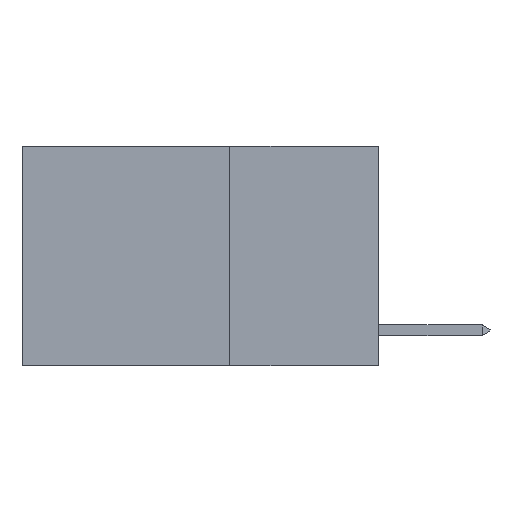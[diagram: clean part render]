
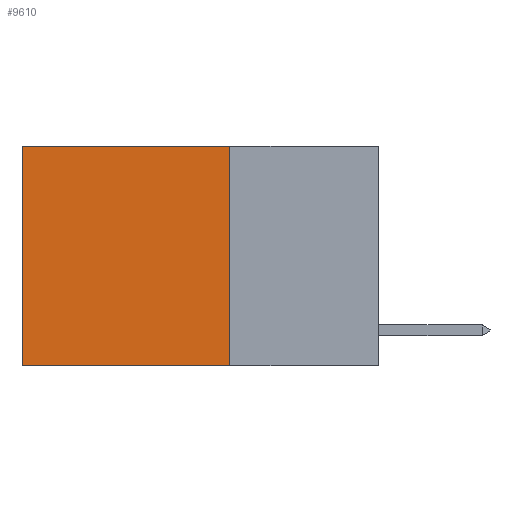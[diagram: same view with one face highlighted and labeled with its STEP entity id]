
A CAD part, left-side view. The second image highlights one B-rep face of the part: STEP entity #9610.
In plain terms, the highlighted planar face has unit normal (-1, 0, 0).
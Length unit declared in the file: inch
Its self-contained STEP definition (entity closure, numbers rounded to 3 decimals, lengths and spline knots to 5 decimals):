
#3048 = CARTESIAN_POINT ( 'NONE',  ( 0.2625, 0.6, -0.37 ) ) ;
#3465 = VECTOR ( 'NONE', #12344, 39.37008 ) ;
#3914 = CARTESIAN_POINT ( 'NONE',  ( 0.2625, 0.25, -0.37 ) ) ;
#4142 = EDGE_CURVE ( 'NONE', #28734, #22519, #23128, .T. ) ;
#4791 = DIRECTION ( 'NONE',  ( 0., 1., 0. ) ) ;
#5929 = CARTESIAN_POINT ( 'NONE',  ( 0.2625, 0.25, 0. ) ) ;
#8169 = VECTOR ( 'NONE', #30940, 39.37008 ) ;
#8349 = DIRECTION ( 'NONE',  ( 0., 0., -1. ) ) ;
#8945 = LINE ( 'NONE', #26161, #8169 ) ;
#9506 = VERTEX_POINT ( 'NONE', #3048 ) ;
#9610 = ADVANCED_FACE ( 'NONE', ( #30795 ), #17893, .F. ) ;
#9884 = LINE ( 'NONE', #14764, #3465 ) ;
#10461 = AXIS2_PLACEMENT_3D ( 'NONE', #5929, #22759, #8349 ) ;
#12344 = DIRECTION ( 'NONE',  ( 0., 0., -1. ) ) ;
#12911 = ORIENTED_EDGE ( 'NONE', *, *, #28765, .T. ) ;
#13564 = EDGE_CURVE ( 'NONE', #29438, #9506, #20241, .T. ) ;
#14479 = CARTESIAN_POINT ( 'NONE',  ( 0.2625, 0.25, -0.37 ) ) ;
#14650 = DIRECTION ( 'NONE',  ( 0., 1., 0. ) ) ;
#14764 = CARTESIAN_POINT ( 'NONE',  ( 0.2625, 0.6, 0. ) ) ;
#15971 = VECTOR ( 'NONE', #14650, 39.37008 ) ;
#17893 = PLANE ( 'NONE',  #10461 ) ;
#17933 = ORIENTED_EDGE ( 'NONE', *, *, #4142, .T. ) ;
#18714 = VECTOR ( 'NONE', #4791, 39.37008 ) ;
#19484 = CARTESIAN_POINT ( 'NONE',  ( 0.2625, 0.25, 0. ) ) ;
#19889 = CARTESIAN_POINT ( 'NONE',  ( 0.2625, 0.6, 0. ) ) ;
#20241 = LINE ( 'NONE', #14479, #18714 ) ;
#22519 = VERTEX_POINT ( 'NONE', #19889 ) ;
#22759 = DIRECTION ( 'NONE',  ( 1., 0., 0. ) ) ;
#23128 = LINE ( 'NONE', #26630, #15971 ) ;
#25168 = ORIENTED_EDGE ( 'NONE', *, *, #13564, .F. ) ;
#25484 = EDGE_LOOP ( 'NONE', ( #12911, #25168, #30778, #17933 ) ) ;
#26161 = CARTESIAN_POINT ( 'NONE',  ( 0.2625, 0.25, 0. ) ) ;
#26630 = CARTESIAN_POINT ( 'NONE',  ( 0.2625, 0.25, 0. ) ) ;
#26730 = EDGE_CURVE ( 'NONE', #28734, #29438, #8945, .T. ) ;
#28734 = VERTEX_POINT ( 'NONE', #19484 ) ;
#28765 = EDGE_CURVE ( 'NONE', #22519, #9506, #9884, .T. ) ;
#29438 = VERTEX_POINT ( 'NONE', #3914 ) ;
#30778 = ORIENTED_EDGE ( 'NONE', *, *, #26730, .F. ) ;
#30795 = FACE_OUTER_BOUND ( 'NONE', #25484, .T. ) ;
#30940 = DIRECTION ( 'NONE',  ( 0., 0., -1. ) ) ;
